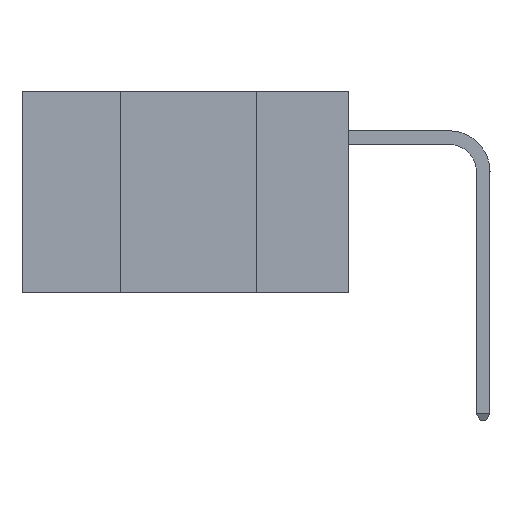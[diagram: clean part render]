
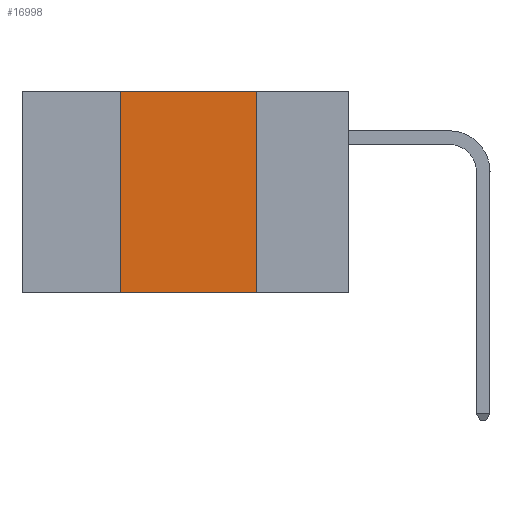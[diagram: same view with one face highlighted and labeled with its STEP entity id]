
A CAD part, left-side view. The second image highlights one B-rep face of the part: STEP entity #16998.
In plain terms, the highlighted planar face has unit normal (-1, 0, 0).
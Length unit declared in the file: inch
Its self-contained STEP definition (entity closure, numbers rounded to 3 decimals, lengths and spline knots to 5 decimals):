
#116 = VECTOR ( 'NONE', #10900, 39.37008 ) ;
#893 = LINE ( 'NONE', #2221, #116 ) ;
#1475 = VERTEX_POINT ( 'NONE', #9686 ) ;
#2221 = CARTESIAN_POINT ( 'NONE',  ( 0., 0.17, 0. ) ) ;
#3307 = VECTOR ( 'NONE', #10554, 39.37008 ) ;
#4829 = CARTESIAN_POINT ( 'NONE',  ( 0., 0.6, 0. ) ) ;
#5169 = LINE ( 'NONE', #9428, #3307 ) ;
#5745 = CARTESIAN_POINT ( 'NONE',  ( 0., 0.6, 0. ) ) ;
#5877 = ORIENTED_EDGE ( 'NONE', *, *, #18631, .F. ) ;
#5913 = CARTESIAN_POINT ( 'NONE',  ( 0., 0.42, -0.37 ) ) ;
#6238 = CARTESIAN_POINT ( 'NONE',  ( 0., 0.17, -0.37 ) ) ;
#6963 = EDGE_LOOP ( 'NONE', ( #10406, #15628, #5877, #16111 ) ) ;
#7255 = DIRECTION ( 'NONE',  ( 0., -1., 0. ) ) ;
#7499 = VERTEX_POINT ( 'NONE', #5913 ) ;
#7756 = LINE ( 'NONE', #15015, #13741 ) ;
#7771 = FACE_OUTER_BOUND ( 'NONE', #6963, .T. ) ;
#8559 = EDGE_CURVE ( 'NONE', #7499, #13114, #5169, .T. ) ;
#8838 = VECTOR ( 'NONE', #7255, 39.37008 ) ;
#8904 = DIRECTION ( 'NONE',  ( 0., 0., -1. ) ) ;
#9428 = CARTESIAN_POINT ( 'NONE',  ( 0., 0.6, -0.37 ) ) ;
#9686 = CARTESIAN_POINT ( 'NONE',  ( 0., 0.17, 0. ) ) ;
#10406 = ORIENTED_EDGE ( 'NONE', *, *, #11115, .F. ) ;
#10429 = EDGE_CURVE ( 'NONE', #14354, #1475, #15658, .T. ) ;
#10554 = DIRECTION ( 'NONE',  ( 0., -1., 0. ) ) ;
#10900 = DIRECTION ( 'NONE',  ( 0., 0., -1. ) ) ;
#11115 = EDGE_CURVE ( 'NONE', #1475, #13114, #893, .T. ) ;
#12232 = AXIS2_PLACEMENT_3D ( 'NONE', #4829, #15030, #8904 ) ;
#12414 = CARTESIAN_POINT ( 'NONE',  ( 0., 0.42, 0. ) ) ;
#13114 = VERTEX_POINT ( 'NONE', #6238 ) ;
#13509 = DIRECTION ( 'NONE',  ( 0., 0., 1. ) ) ;
#13741 = VECTOR ( 'NONE', #13509, 39.37008 ) ;
#14354 = VERTEX_POINT ( 'NONE', #12414 ) ;
#15015 = CARTESIAN_POINT ( 'NONE',  ( 0., 0.42, 0. ) ) ;
#15030 = DIRECTION ( 'NONE',  ( 1., 0., 0. ) ) ;
#15628 = ORIENTED_EDGE ( 'NONE', *, *, #10429, .F. ) ;
#15658 = LINE ( 'NONE', #5745, #8838 ) ;
#16111 = ORIENTED_EDGE ( 'NONE', *, *, #8559, .T. ) ;
#16998 = ADVANCED_FACE ( 'NONE', ( #7771 ), #17758, .F. ) ;
#17758 = PLANE ( 'NONE',  #12232 ) ;
#18631 = EDGE_CURVE ( 'NONE', #7499, #14354, #7756, .T. ) ;
